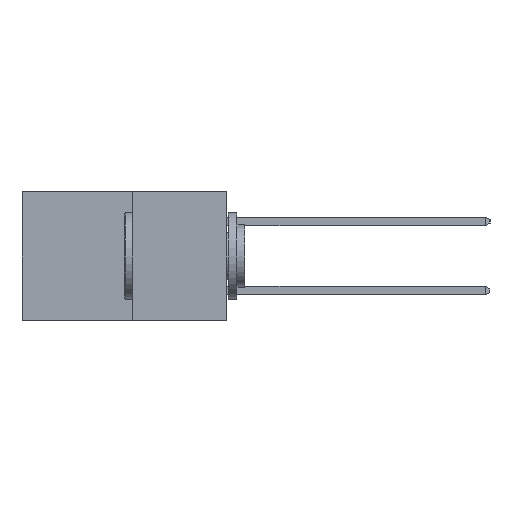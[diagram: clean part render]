
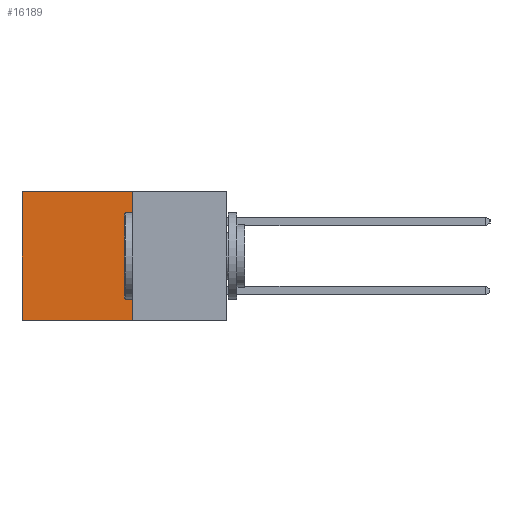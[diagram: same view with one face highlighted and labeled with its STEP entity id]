
A CAD part, left-side view. The second image highlights one B-rep face of the part: STEP entity #16189.
In plain terms, the highlighted planar face has unit normal (-1, 0, 0).
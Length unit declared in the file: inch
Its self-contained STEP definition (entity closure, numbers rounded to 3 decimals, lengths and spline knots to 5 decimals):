
#688 = EDGE_CURVE ( 'NONE', #21116, #10641, #17106, .T. ) ;
#914 = DIRECTION ( 'NONE',  ( 0., 0., -1. ) ) ;
#2617 = LINE ( 'NONE', #14846, #20259 ) ;
#3352 = LINE ( 'NONE', #16513, #12853 ) ;
#3523 = DIRECTION ( 'NONE',  ( 0., 0., -1. ) ) ;
#5327 = CARTESIAN_POINT ( 'NONE',  ( 0.277, 0.27, 0. ) ) ;
#5968 = DIRECTION ( 'NONE',  ( 0., 1., 0. ) ) ;
#6181 = VERTEX_POINT ( 'NONE', #6371 ) ;
#6371 = CARTESIAN_POINT ( 'NONE',  ( 0.277, 0.27, -0.37 ) ) ;
#6670 = FACE_OUTER_BOUND ( 'NONE', #8703, .T. ) ;
#7227 = AXIS2_PLACEMENT_3D ( 'NONE', #11663, #11736, #914 ) ;
#7464 = DIRECTION ( 'NONE',  ( 0., 1., 0. ) ) ;
#8703 = EDGE_LOOP ( 'NONE', ( #21983, #8819, #19390, #14746 ) ) ;
#8819 = ORIENTED_EDGE ( 'NONE', *, *, #8861, .F. ) ;
#8861 = EDGE_CURVE ( 'NONE', #6181, #20820, #3352, .T. ) ;
#9475 = CARTESIAN_POINT ( 'NONE',  ( 0.277, 0.59, 0. ) ) ;
#9588 = VECTOR ( 'NONE', #3523, 39.37008 ) ;
#9962 = PLANE ( 'NONE',  #7227 ) ;
#10641 = VERTEX_POINT ( 'NONE', #9475 ) ;
#11663 = CARTESIAN_POINT ( 'NONE',  ( 0.277, 0.27, -0.37 ) ) ;
#11674 = CARTESIAN_POINT ( 'NONE',  ( 0.277, 0.59, -0.37 ) ) ;
#11736 = DIRECTION ( 'NONE',  ( 1., 0., 0. ) ) ;
#12447 = CARTESIAN_POINT ( 'NONE',  ( 0.277, 0.59, -0.37 ) ) ;
#12472 = VECTOR ( 'NONE', #7464, 39.37008 ) ;
#12760 = CARTESIAN_POINT ( 'NONE',  ( 0.277, 0.27, 0. ) ) ;
#12853 = VECTOR ( 'NONE', #5968, 39.37008 ) ;
#14746 = ORIENTED_EDGE ( 'NONE', *, *, #688, .T. ) ;
#14846 = CARTESIAN_POINT ( 'NONE',  ( 0.277, 0.27, -0.37 ) ) ;
#16189 = ADVANCED_FACE ( 'NONE', ( #6670 ), #9962, .F. ) ;
#16513 = CARTESIAN_POINT ( 'NONE',  ( 0.277, 0.27, -0.37 ) ) ;
#17106 = LINE ( 'NONE', #12760, #12472 ) ;
#17392 = EDGE_CURVE ( 'NONE', #21116, #6181, #2617, .T. ) ;
#19390 = ORIENTED_EDGE ( 'NONE', *, *, #17392, .F. ) ;
#19877 = LINE ( 'NONE', #12447, #9588 ) ;
#20044 = DIRECTION ( 'NONE',  ( 0., 0., -1. ) ) ;
#20259 = VECTOR ( 'NONE', #20044, 39.37008 ) ;
#20820 = VERTEX_POINT ( 'NONE', #11674 ) ;
#21116 = VERTEX_POINT ( 'NONE', #5327 ) ;
#21801 = EDGE_CURVE ( 'NONE', #10641, #20820, #19877, .T. ) ;
#21983 = ORIENTED_EDGE ( 'NONE', *, *, #21801, .T. ) ;
